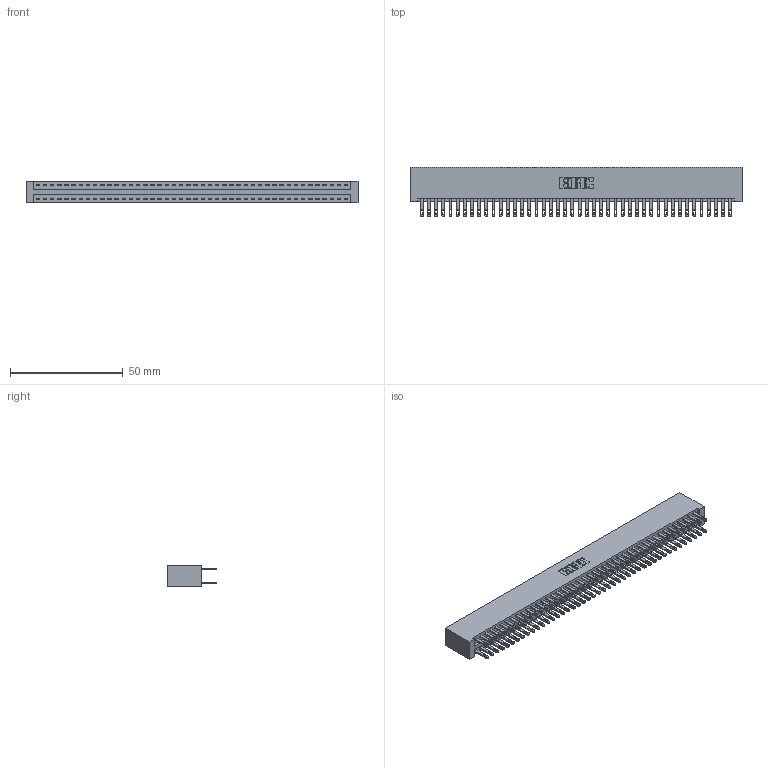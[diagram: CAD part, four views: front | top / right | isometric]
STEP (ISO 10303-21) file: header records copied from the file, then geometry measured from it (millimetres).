
FILE_DESCRIPTION (( 'STEP AP203' ), '1' );
FILE_NAME ('346-088-500-201.STEP', '2018-08-29T23:34:23', ( '' ), ( '' ), 'SwSTEP 2.0', 'SolidWorks 2016', '' );
FILE_SCHEMA (( 'CONFIG_CONTROL_DESIGN' ));
Length unit declared in the file: inch
Products named in the file (3): 346 Part_No Mounting Lugs; 345-292-001_345-293-100; 346-088-500-201
Assembly tree (89 placements, depth 2):
  346-088-500-201
    346 Part_No Mounting Lugs
    345-292-001_345-293-100  x88
Bounding box: 146.94 x 21.84 x 9.4 mm (x, y, z)
Volume: 15186.1 mm3; surface area: 21990 mm2
Topology: 89 solids, 89 shells, 4338 faces, 13241 edges, 8826 vertices
Faces by surface type: plane 2624, cylinder 1714
Entity records: 28099 total; most frequent: CARTESIAN_POINT 4624, ORIENTED_EDGE 4558, DIRECTION 4123, EDGE_CURVE 2279, LINE 1975, VECTOR 1975, VERTEX_POINT 1518, AXIS2_PLACEMENT_3D 1074
